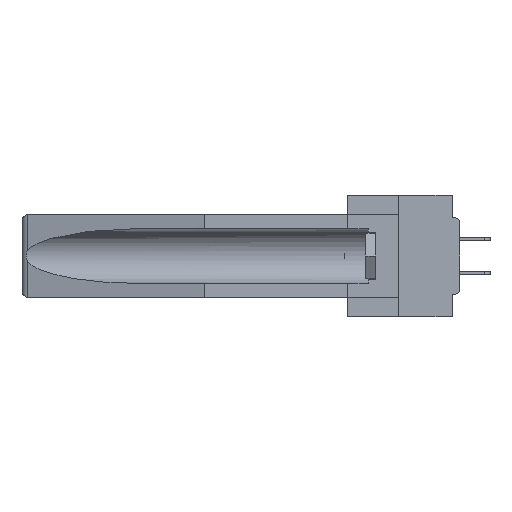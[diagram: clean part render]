
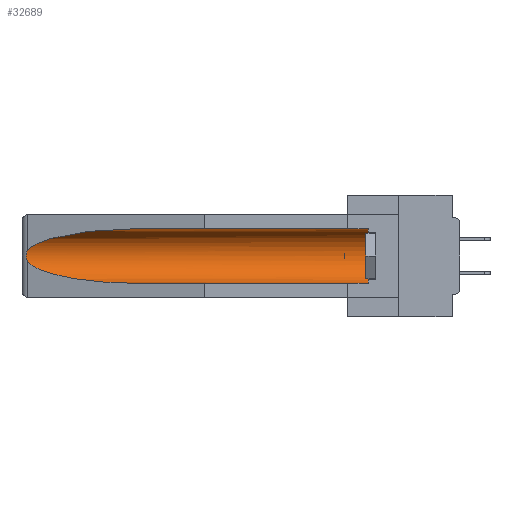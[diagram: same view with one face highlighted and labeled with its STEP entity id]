
A CAD part, left-side view. The second image highlights one B-rep face of the part: STEP entity #32689.
In plain terms, the highlighted cylindrical face has radius 2.857 mm (diameter 5.715 mm), a partial arc.
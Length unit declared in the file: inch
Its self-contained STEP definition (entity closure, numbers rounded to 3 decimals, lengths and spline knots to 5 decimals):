
#503 = B_SPLINE_CURVE_WITH_KNOTS ( 'NONE', 3,
 ( #34585, #19382, #23864, #45738, #1352, #4329, #30628, #23208, #12003, #38362 ),
 .UNSPECIFIED., .F., .F.,
 ( 4, 2, 2, 2, 4 ),
 ( 0., 0.00029, 0.00058, 0.00087, 0.00117 ),
 .UNSPECIFIED. ) ;
#1352 = CARTESIAN_POINT ( 'NONE',  ( 0.2675, 1.53308, -0.16763 ) ) ;
#1973 = CARTESIAN_POINT ( 'NONE',  ( 0.26537, 1.52718, -0.19328 ) ) ;
#2130 = CYLINDRICAL_SURFACE ( 'NONE', #7502, 0.1125 ) ;
#3624 = EDGE_LOOP ( 'NONE', ( #23731, #26466, #11722, #31943, #17750, #26178 ) ) ;
#4329 = CARTESIAN_POINT ( 'NONE',  ( 0.2675, 1.53308, -0.17534 ) ) ;
#5550 = LINE ( 'NONE', #12746, #13686 ) ;
#7502 = AXIS2_PLACEMENT_3D ( 'NONE', #20943, #20770, #13682 ) ;
#9766 = FACE_OUTER_BOUND ( 'NONE', #3624, .T. ) ;
#11722 = ORIENTED_EDGE ( 'NONE', *, *, #29599, .T. ) ;
#12003 = CARTESIAN_POINT ( 'NONE',  ( 0.26597, 1.5296, -0.19026 ) ) ;
#12053 = CARTESIAN_POINT ( 'NONE',  ( 0.155, 1.07973, -0.059 ) ) ;
#12210 =( BOUNDED_CURVE ( )  B_SPLINE_CURVE ( 3, ( #12053, #45782, #45948, #22937 ),
 .UNSPECIFIED., .F., .T. ) 
 B_SPLINE_CURVE_WITH_KNOTS ( ( 4, 4 ),
 ( 4.71239, 6.08839 ),
 .UNSPECIFIED. ) 
 CURVE ( )  GEOMETRIC_REPRESENTATION_ITEM ( )  RATIONAL_B_SPLINE_CURVE ( ( 1., 0.848, 0.848, 1. ) ) 
 REPRESENTATION_ITEM ( '' )  );
#12746 = CARTESIAN_POINT ( 'NONE',  ( 0.155, -0.30754, -0.059 ) ) ;
#12787 = CARTESIAN_POINT ( 'NONE',  ( 0.25451, 1.48313, -0.24835 ) ) ;
#13339 = CARTESIAN_POINT ( 'NONE',  ( 0.155, 1.07973, -0.059 ) ) ;
#13682 = DIRECTION ( 'NONE',  ( 0., 0., 1. ) ) ;
#13686 = VECTOR ( 'NONE', #16527, 39.37008 ) ;
#14478 = CIRCLE ( 'NONE', #35899, 0.1125 ) ;
#14822 = CARTESIAN_POINT ( 'NONE',  ( 0.155, 0.126, -0.059 ) ) ;
#16407 = CARTESIAN_POINT ( 'NONE',  ( 0.155, -0.30754, -0.284 ) ) ;
#16527 = DIRECTION ( 'NONE',  ( 0., 1., 0. ) ) ;
#16897 = CARTESIAN_POINT ( 'NONE',  ( 0.21114, 1.30732, -0.284 ) ) ;
#17098 = EDGE_CURVE ( 'NONE', #41756, #39307, #5550, .T. ) ;
#17169 = VERTEX_POINT ( 'NONE', #42483 ) ;
#17750 = ORIENTED_EDGE ( 'NONE', *, *, #23282, .T. ) ;
#18890 = VERTEX_POINT ( 'NONE', #32259 ) ;
#19382 = CARTESIAN_POINT ( 'NONE',  ( 0.26597, 1.52961, -0.15275 ) ) ;
#19436 = EDGE_CURVE ( 'NONE', #29222, #18890, #23480, .T. ) ;
#20695 = CARTESIAN_POINT ( 'NONE',  ( 0.155, 1.07973, -0.284 ) ) ;
#20770 = DIRECTION ( 'NONE',  ( 0., 1., 0. ) ) ;
#20943 = CARTESIAN_POINT ( 'NONE',  ( 0.155, -0.30754, -0.1715 ) ) ;
#22937 = CARTESIAN_POINT ( 'NONE',  ( 0.26537, 1.52718, -0.14972 ) ) ;
#23208 = CARTESIAN_POINT ( 'NONE',  ( 0.26655, 1.53094, -0.18657 ) ) ;
#23282 = EDGE_CURVE ( 'NONE', #29222, #41756, #14478, .T. ) ;
#23480 = LINE ( 'NONE', #16407, #35897 ) ;
#23731 = ORIENTED_EDGE ( 'NONE', *, *, #38655, .T. ) ;
#23864 = CARTESIAN_POINT ( 'NONE',  ( 0.26654, 1.53092, -0.15636 ) ) ;
#26178 = ORIENTED_EDGE ( 'NONE', *, *, #17098, .T. ) ;
#26466 = ORIENTED_EDGE ( 'NONE', *, *, #32893, .T. ) ;
#27317 = DIRECTION ( 'NONE',  ( 0., 1., 0. ) ) ;
#29222 = VERTEX_POINT ( 'NONE', #32765 ) ;
#29599 = EDGE_CURVE ( 'NONE', #30910, #18890, #33358, .T. ) ;
#30572 = DIRECTION ( 'NONE',  ( 0., -1., 0. ) ) ;
#30628 = CARTESIAN_POINT ( 'NONE',  ( 0.2673, 1.53269, -0.17917 ) ) ;
#30910 = VERTEX_POINT ( 'NONE', #44166 ) ;
#31943 = ORIENTED_EDGE ( 'NONE', *, *, #19436, .F. ) ;
#32259 = CARTESIAN_POINT ( 'NONE',  ( 0.155, 1.07973, -0.284 ) ) ;
#32689 = ADVANCED_FACE ( 'NONE', ( #9766 ), #2130, .F. ) ;
#32765 = CARTESIAN_POINT ( 'NONE',  ( 0.155, 0.126, -0.284 ) ) ;
#32893 = EDGE_CURVE ( 'NONE', #17169, #30910, #503, .T. ) ;
#33358 =( BOUNDED_CURVE ( )  B_SPLINE_CURVE ( 3, ( #1973, #12787, #16897, #20695 ),
 .UNSPECIFIED., .F., .F. ) 
 B_SPLINE_CURVE_WITH_KNOTS ( ( 4, 4 ),
 ( 0.1948, 1.5708 ),
 .UNSPECIFIED. ) 
 CURVE ( )  GEOMETRIC_REPRESENTATION_ITEM ( )  RATIONAL_B_SPLINE_CURVE ( ( 1., 0.848, 0.848, 1. ) ) 
 REPRESENTATION_ITEM ( '' )  );
#34207 = CARTESIAN_POINT ( 'NONE',  ( 0.155, 0.126, -0.1715 ) ) ;
#34585 = CARTESIAN_POINT ( 'NONE',  ( 0.26537, 1.52718, -0.14972 ) ) ;
#35897 = VECTOR ( 'NONE', #27317, 39.37008 ) ;
#35899 = AXIS2_PLACEMENT_3D ( 'NONE', #34207, #30572, #37666 ) ;
#37666 = DIRECTION ( 'NONE',  ( 0., 0., 1. ) ) ;
#38362 = CARTESIAN_POINT ( 'NONE',  ( 0.26537, 1.52718, -0.19328 ) ) ;
#38655 = EDGE_CURVE ( 'NONE', #39307, #17169, #12210, .T. ) ;
#39307 = VERTEX_POINT ( 'NONE', #13339 ) ;
#41756 = VERTEX_POINT ( 'NONE', #14822 ) ;
#42483 = CARTESIAN_POINT ( 'NONE',  ( 0.26537, 1.52718, -0.14972 ) ) ;
#44166 = CARTESIAN_POINT ( 'NONE',  ( 0.26537, 1.52718, -0.19328 ) ) ;
#45738 = CARTESIAN_POINT ( 'NONE',  ( 0.2673, 1.5327, -0.16383 ) ) ;
#45782 = CARTESIAN_POINT ( 'NONE',  ( 0.21114, 1.30732, -0.059 ) ) ;
#45948 = CARTESIAN_POINT ( 'NONE',  ( 0.25451, 1.48313, -0.09465 ) ) ;
